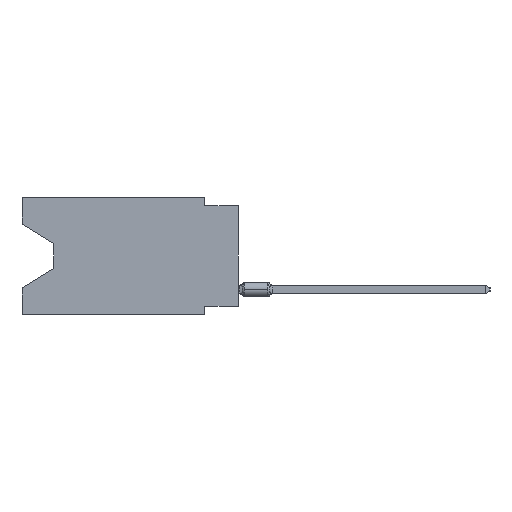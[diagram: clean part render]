
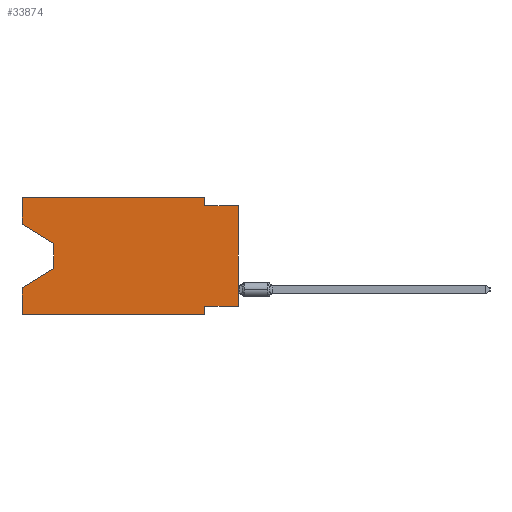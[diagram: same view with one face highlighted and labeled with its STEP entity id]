
A CAD part, left-side view. The second image highlights one B-rep face of the part: STEP entity #33874.
In plain terms, the highlighted planar face has unit normal (-1, 0, 0).
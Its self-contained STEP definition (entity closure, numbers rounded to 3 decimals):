
#736 = VERTEX_POINT ( 'NONE', #22272 ) ;
#853 = LINE ( 'NONE', #29768, #23673 ) ;
#1042 = LINE ( 'NONE', #47995, #40501 ) ;
#1346 = VERTEX_POINT ( 'NONE', #49148 ) ;
#2844 = FACE_OUTER_BOUND ( 'NONE', #45587, .T. ) ;
#3751 = CARTESIAN_POINT ( 'NONE',  ( 0., 13.97, -3.505 ) ) ;
#3946 = VERTEX_POINT ( 'NONE', #57308 ) ;
#5004 = VERTEX_POINT ( 'NONE', #41882 ) ;
#5358 = DIRECTION ( 'NONE',  ( 0., -0.855, -0.519 ) ) ;
#6484 = CARTESIAN_POINT ( 'NONE',  ( 0., 16.383, 0. ) ) ;
#6485 = DIRECTION ( 'NONE',  ( 0., 0., 1. ) ) ;
#7239 = DIRECTION ( 'NONE',  ( 0., 0., -1. ) ) ;
#7942 = EDGE_CURVE ( 'NONE', #8887, #33656, #29141, .T. ) ;
#8857 = VECTOR ( 'NONE', #44921, 1000. ) ;
#8887 = VERTEX_POINT ( 'NONE', #23740 ) ;
#9054 = DIRECTION ( 'NONE',  ( 0., 0., -1. ) ) ;
#10206 = ORIENTED_EDGE ( 'NONE', *, *, #16077, .T. ) ;
#11093 = LINE ( 'NONE', #53642, #48406 ) ;
#11288 = ORIENTED_EDGE ( 'NONE', *, *, #39668, .T. ) ;
#11430 = EDGE_CURVE ( 'NONE', #736, #11794, #21203, .T. ) ;
#11474 = LINE ( 'NONE', #21729, #29413 ) ;
#11546 = DIRECTION ( 'NONE',  ( 0., 0., 1. ) ) ;
#11794 = VERTEX_POINT ( 'NONE', #6484 ) ;
#11826 = LINE ( 'NONE', #58105, #38119 ) ;
#12658 = CARTESIAN_POINT ( 'NONE',  ( 0., 2.54, -8.89 ) ) ;
#12705 = VECTOR ( 'NONE', #20774, 1000. ) ;
#13964 = ORIENTED_EDGE ( 'NONE', *, *, #54575, .T. ) ;
#14553 = EDGE_CURVE ( 'NONE', #50489, #8887, #1042, .T. ) ;
#15222 = CARTESIAN_POINT ( 'NONE',  ( 0., 2.54, 0. ) ) ;
#15442 = VECTOR ( 'NONE', #61422, 1000. ) ;
#16077 = EDGE_CURVE ( 'NONE', #50293, #33656, #58574, .T. ) ;
#16450 = DIRECTION ( 'NONE',  ( 0., -1., 0. ) ) ;
#16931 = EDGE_CURVE ( 'NONE', #50489, #24019, #53716, .T. ) ;
#17183 = PLANE ( 'NONE',  #35213 ) ;
#18708 = VERTEX_POINT ( 'NONE', #15222 ) ;
#19072 = ORIENTED_EDGE ( 'NONE', *, *, #14553, .F. ) ;
#20774 = DIRECTION ( 'NONE',  ( 0., -1., 0. ) ) ;
#21203 = LINE ( 'NONE', #39800, #41426 ) ;
#21729 = CARTESIAN_POINT ( 'NONE',  ( 0., 16.383, 0. ) ) ;
#22272 = CARTESIAN_POINT ( 'NONE',  ( 0., 16.383, -2.038 ) ) ;
#23593 = LINE ( 'NONE', #33193, #12705 ) ;
#23673 = VECTOR ( 'NONE', #38773, 1000. ) ;
#23740 = CARTESIAN_POINT ( 'NONE',  ( 0., 2.54, -8.255 ) ) ;
#24019 = VERTEX_POINT ( 'NONE', #33777 ) ;
#24454 = VECTOR ( 'NONE', #5358, 1000. ) ;
#25211 = DIRECTION ( 'NONE',  ( 0., 0., -1. ) ) ;
#27400 = LINE ( 'NONE', #3751, #41045 ) ;
#29141 = LINE ( 'NONE', #47469, #15442 ) ;
#29413 = VECTOR ( 'NONE', #16450, 1000. ) ;
#29768 = CARTESIAN_POINT ( 'NONE',  ( 0., 16.383, 0. ) ) ;
#29887 = ORIENTED_EDGE ( 'NONE', *, *, #58289, .T. ) ;
#30266 = ORIENTED_EDGE ( 'NONE', *, *, #37106, .F. ) ;
#31353 = EDGE_CURVE ( 'NONE', #18708, #3946, #11826, .T. ) ;
#31759 = CARTESIAN_POINT ( 'NONE',  ( 0., 16.383, 0. ) ) ;
#32762 = CARTESIAN_POINT ( 'NONE',  ( 0., 16.383, -6.852 ) ) ;
#33193 = CARTESIAN_POINT ( 'NONE',  ( 0., 0., -0.635 ) ) ;
#33656 = VERTEX_POINT ( 'NONE', #12658 ) ;
#33777 = CARTESIAN_POINT ( 'NONE',  ( 0., 0., -0.635 ) ) ;
#33874 = ADVANCED_FACE ( 'NONE', ( #2844 ), #17183, .F. ) ;
#34232 = ORIENTED_EDGE ( 'NONE', *, *, #39319, .F. ) ;
#35213 = AXIS2_PLACEMENT_3D ( 'NONE', #31759, #41070, #7239 ) ;
#36994 = EDGE_CURVE ( 'NONE', #3946, #24019, #23593, .T. ) ;
#37106 = EDGE_CURVE ( 'NONE', #50293, #49041, #853, .T. ) ;
#38119 = VECTOR ( 'NONE', #25211, 1000. ) ;
#38773 = DIRECTION ( 'NONE',  ( 0., 0., 1. ) ) ;
#39319 = EDGE_CURVE ( 'NONE', #11794, #18708, #11474, .T. ) ;
#39668 = EDGE_CURVE ( 'NONE', #5004, #49041, #11093, .T. ) ;
#39800 = CARTESIAN_POINT ( 'NONE',  ( 0., 16.383, 0. ) ) ;
#40501 = VECTOR ( 'NONE', #52949, 1000. ) ;
#40836 = ORIENTED_EDGE ( 'NONE', *, *, #11430, .F. ) ;
#41045 = VECTOR ( 'NONE', #9054, 1000. ) ;
#41070 = DIRECTION ( 'NONE',  ( 1., 0., 0. ) ) ;
#41426 = VECTOR ( 'NONE', #11546, 1000. ) ;
#41882 = CARTESIAN_POINT ( 'NONE',  ( 0., 13.97, -5.385 ) ) ;
#42417 = ORIENTED_EDGE ( 'NONE', *, *, #16931, .T. ) ;
#42604 = CARTESIAN_POINT ( 'NONE',  ( 0., 0., -8.255 ) ) ;
#44921 = DIRECTION ( 'NONE',  ( 0., -1., 0. ) ) ;
#45587 = EDGE_LOOP ( 'NONE', ( #29887, #13964, #11288, #30266, #10206, #56588, #19072, #42417, #60768, #47693, #34232, #40836 ) ) ;
#47469 = CARTESIAN_POINT ( 'NONE',  ( 0., 2.54, -8.89 ) ) ;
#47693 = ORIENTED_EDGE ( 'NONE', *, *, #31353, .F. ) ;
#47995 = CARTESIAN_POINT ( 'NONE',  ( 0., 0., -8.255 ) ) ;
#48406 = VECTOR ( 'NONE', #54549, 1000. ) ;
#48844 = CARTESIAN_POINT ( 'NONE',  ( 0., 16.383, -2.038 ) ) ;
#49041 = VERTEX_POINT ( 'NONE', #32762 ) ;
#49053 = CARTESIAN_POINT ( 'NONE',  ( 0., 0., 0. ) ) ;
#49148 = CARTESIAN_POINT ( 'NONE',  ( 0., 13.97, -3.505 ) ) ;
#50293 = VERTEX_POINT ( 'NONE', #55224 ) ;
#50489 = VERTEX_POINT ( 'NONE', #42604 ) ;
#52949 = DIRECTION ( 'NONE',  ( 0., 1., 0. ) ) ;
#53322 = CARTESIAN_POINT ( 'NONE',  ( 0., 16.383, -8.89 ) ) ;
#53642 = CARTESIAN_POINT ( 'NONE',  ( 0., 13.97, -5.385 ) ) ;
#53716 = LINE ( 'NONE', #49053, #57396 ) ;
#54549 = DIRECTION ( 'NONE',  ( 0., 0.855, -0.519 ) ) ;
#54575 = EDGE_CURVE ( 'NONE', #1346, #5004, #27400, .T. ) ;
#55224 = CARTESIAN_POINT ( 'NONE',  ( 0., 16.383, -8.89 ) ) ;
#56588 = ORIENTED_EDGE ( 'NONE', *, *, #7942, .F. ) ;
#56924 = LINE ( 'NONE', #48844, #24454 ) ;
#57308 = CARTESIAN_POINT ( 'NONE',  ( 0., 2.54, -0.635 ) ) ;
#57396 = VECTOR ( 'NONE', #6485, 1000. ) ;
#58105 = CARTESIAN_POINT ( 'NONE',  ( 0., 2.54, 0. ) ) ;
#58289 = EDGE_CURVE ( 'NONE', #736, #1346, #56924, .T. ) ;
#58574 = LINE ( 'NONE', #53322, #8857 ) ;
#60768 = ORIENTED_EDGE ( 'NONE', *, *, #36994, .F. ) ;
#61422 = DIRECTION ( 'NONE',  ( 0., 0., -1. ) ) ;
